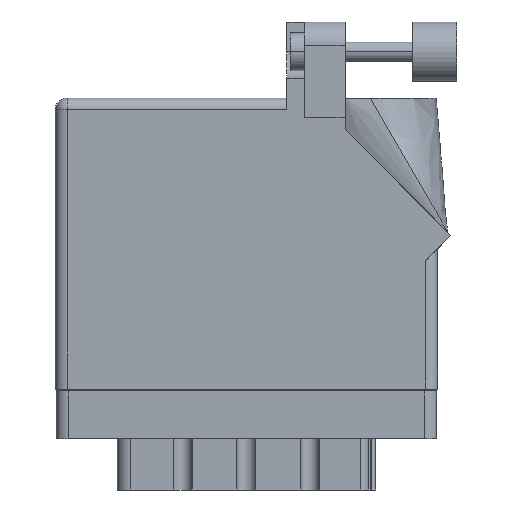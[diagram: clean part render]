
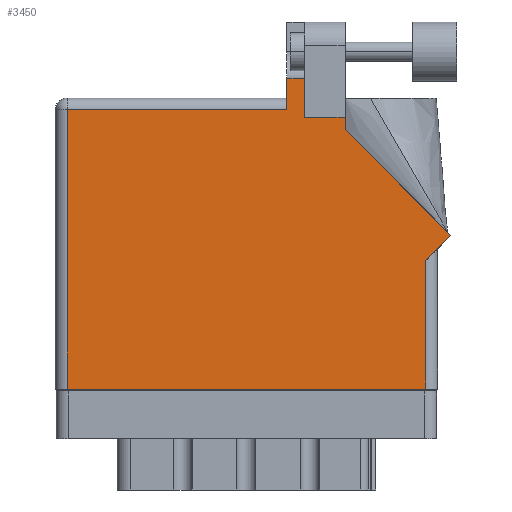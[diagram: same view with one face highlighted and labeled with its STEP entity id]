
A CAD part, front view. The second image highlights one B-rep face of the part: STEP entity #3450.
In plain terms, the highlighted face is planar.
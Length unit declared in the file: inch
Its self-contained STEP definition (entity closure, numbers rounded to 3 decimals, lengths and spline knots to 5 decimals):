
#1337 = CARTESIAN_POINT ( 'NONE',  ( 2.01, 0.737, 0. ) ) ;
#1990 = DIRECTION ( 'NONE',  ( 0., 0., -1. ) ) ;
#2199 = DIRECTION ( 'NONE',  ( 0., 1., 0. ) ) ;
#2645 = CARTESIAN_POINT ( 'NONE',  ( 1.311, 1.43, 0. ) ) ;
#2704 = VERTEX_POINT ( 'NONE', #9320 ) ;
#3338 = VECTOR ( 'NONE', #2199, 39.37008 ) ;
#3450 = ADVANCED_FACE ( 'NONE', ( #28694 ), #10248, .F. ) ;
#3927 = ORIENTED_EDGE ( 'NONE', *, *, #25449, .T. ) ;
#4566 = CARTESIAN_POINT ( 'NONE',  ( 1.311, 1.43, 0. ) ) ;
#4625 = LINE ( 'NONE', #37201, #21853 ) ;
#4755 = DIRECTION ( 'NONE',  ( -1., 0., 0. ) ) ;
#4997 = CARTESIAN_POINT ( 'NONE',  ( 1.524, 1.36442, 0. ) ) ;
#5608 = VERTEX_POINT ( 'NONE', #6258 ) ;
#6083 = EDGE_CURVE ( 'NONE', #9348, #12156, #30414, .T. ) ;
#6258 = CARTESIAN_POINT ( 'NONE',  ( 1.948, 0.675, 0. ) ) ;
#6453 = ORIENTED_EDGE ( 'NONE', *, *, #9667, .T. ) ;
#6529 = DIRECTION ( 'NONE',  ( 0., -1., 0. ) ) ;
#6634 = CARTESIAN_POINT ( 'NONE',  ( 1.524, 1.36442, 0. ) ) ;
#7300 = AXIS2_PLACEMENT_3D ( 'NONE', #19517, #1990, #31050 ) ;
#7605 = LINE ( 'NONE', #36098, #27580 ) ;
#7659 = CARTESIAN_POINT ( 'NONE',  ( 0., 1.468, 0. ) ) ;
#7669 = LINE ( 'NONE', #35610, #36247 ) ;
#8087 = ORIENTED_EDGE ( 'NONE', *, *, #18436, .T. ) ;
#8394 = CARTESIAN_POINT ( 'NONE',  ( 2.08071, 0.80771, 0. ) ) ;
#8496 = CARTESIAN_POINT ( 'NONE',  ( 1.217, 1.468, 0. ) ) ;
#9320 = CARTESIAN_POINT ( 'NONE',  ( 0.062, 1.468, 0. ) ) ;
#9348 = VERTEX_POINT ( 'NONE', #31632 ) ;
#9414 = CARTESIAN_POINT ( 'NONE',  ( 1.948, 0., 0. ) ) ;
#9667 = EDGE_CURVE ( 'NONE', #27981, #18224, #4625, .T. ) ;
#9725 = DIRECTION ( 'NONE',  ( 1., 0., 0. ) ) ;
#9809 = VERTEX_POINT ( 'NONE', #14018 ) ;
#9871 = DIRECTION ( 'NONE',  ( 0.707, 0.707, 0. ) ) ;
#10069 = ORIENTED_EDGE ( 'NONE', *, *, #20726, .T. ) ;
#10248 = PLANE ( 'NONE',  #7300 ) ;
#12108 = LINE ( 'NONE', #33736, #21128 ) ;
#12156 = VERTEX_POINT ( 'NONE', #6634 ) ;
#12233 = VERTEX_POINT ( 'NONE', #9414 ) ;
#12441 = VECTOR ( 'NONE', #34024, 39.37008 ) ;
#13345 = LINE ( 'NONE', #7659, #12441 ) ;
#14018 = CARTESIAN_POINT ( 'NONE',  ( 1.524, 1.43, 0. ) ) ;
#14030 = ORIENTED_EDGE ( 'NONE', *, *, #32396, .T. ) ;
#14276 = LINE ( 'NONE', #22393, #21044 ) ;
#15120 = CARTESIAN_POINT ( 'NONE',  ( 1.217, 1.6315, 0. ) ) ;
#16359 = DIRECTION ( 'NONE',  ( 0., 1., 0. ) ) ;
#16411 = EDGE_CURVE ( 'NONE', #22450, #12233, #32789, .T. ) ;
#18224 = VERTEX_POINT ( 'NONE', #8496 ) ;
#18436 = EDGE_CURVE ( 'NONE', #27429, #27981, #7669, .T. ) ;
#19517 = CARTESIAN_POINT ( 'NONE',  ( 0., 1.53, 0. ) ) ;
#19787 = DIRECTION ( 'NONE',  ( 0., 1., 0. ) ) ;
#20041 = DIRECTION ( 'NONE',  ( 0., -1., 0. ) ) ;
#20726 = EDGE_CURVE ( 'NONE', #2704, #22450, #7605, .T. ) ;
#21044 = VECTOR ( 'NONE', #22137, 39.37008 ) ;
#21128 = VECTOR ( 'NONE', #16359, 39.37008 ) ;
#21853 = VECTOR ( 'NONE', #20041, 39.37008 ) ;
#22137 = DIRECTION ( 'NONE',  ( -1., 0., 0. ) ) ;
#22393 = CARTESIAN_POINT ( 'NONE',  ( 1.524, 1.43, 0. ) ) ;
#22450 = VERTEX_POINT ( 'NONE', #26945 ) ;
#22606 = DIRECTION ( 'NONE',  ( -0.707, 0.707, 0. ) ) ;
#23024 = VECTOR ( 'NONE', #9871, 39.37008 ) ;
#23461 = LINE ( 'NONE', #1337, #23024 ) ;
#23972 = ORIENTED_EDGE ( 'NONE', *, *, #24792, .T. ) ;
#24242 = LINE ( 'NONE', #4997, #3338 ) ;
#24792 = EDGE_CURVE ( 'NONE', #12233, #5608, #12108, .T. ) ;
#25449 = EDGE_CURVE ( 'NONE', #12156, #9809, #24242, .T. ) ;
#25492 = ORIENTED_EDGE ( 'NONE', *, *, #16411, .T. ) ;
#25584 = ORIENTED_EDGE ( 'NONE', *, *, #29218, .T. ) ;
#25843 = VERTEX_POINT ( 'NONE', #4566 ) ;
#26328 = CARTESIAN_POINT ( 'NONE',  ( 1.311, 1.6315, 0. ) ) ;
#26468 = VECTOR ( 'NONE', #9725, 39.37008 ) ;
#26716 = ORIENTED_EDGE ( 'NONE', *, *, #31774, .T. ) ;
#26945 = CARTESIAN_POINT ( 'NONE',  ( 0.062, 0., 0. ) ) ;
#27258 = ORIENTED_EDGE ( 'NONE', *, *, #6083, .T. ) ;
#27429 = VERTEX_POINT ( 'NONE', #26328 ) ;
#27580 = VECTOR ( 'NONE', #6529, 39.37008 ) ;
#27981 = VERTEX_POINT ( 'NONE', #15120 ) ;
#28694 = FACE_OUTER_BOUND ( 'NONE', #32839, .T. ) ;
#29218 = EDGE_CURVE ( 'NONE', #5608, #9348, #23461, .T. ) ;
#30400 = CARTESIAN_POINT ( 'NONE',  ( 0., 0., 0. ) ) ;
#30414 = LINE ( 'NONE', #8394, #36334 ) ;
#31050 = DIRECTION ( 'NONE',  ( -1., 0., 0. ) ) ;
#31632 = CARTESIAN_POINT ( 'NONE',  ( 2.08071, 0.80771, 0. ) ) ;
#31774 = EDGE_CURVE ( 'NONE', #18224, #2704, #13345, .T. ) ;
#32304 = ORIENTED_EDGE ( 'NONE', *, *, #34923, .T. ) ;
#32396 = EDGE_CURVE ( 'NONE', #25843, #27429, #37551, .T. ) ;
#32789 = LINE ( 'NONE', #30400, #26468 ) ;
#32839 = EDGE_LOOP ( 'NONE', ( #14030, #8087, #6453, #26716, #10069, #25492, #23972, #25584, #27258, #3927, #32304 ) ) ;
#33736 = CARTESIAN_POINT ( 'NONE',  ( 1.948, 0.737, 0. ) ) ;
#34024 = DIRECTION ( 'NONE',  ( -1., 0., 0. ) ) ;
#34923 = EDGE_CURVE ( 'NONE', #9809, #25843, #14276, .T. ) ;
#35610 = CARTESIAN_POINT ( 'NONE',  ( 1.64177, 1.6315, 0. ) ) ;
#36098 = CARTESIAN_POINT ( 'NONE',  ( 0.062, 0., 0. ) ) ;
#36186 = VECTOR ( 'NONE', #19787, 39.37008 ) ;
#36247 = VECTOR ( 'NONE', #4755, 39.37008 ) ;
#36334 = VECTOR ( 'NONE', #22606, 39.37008 ) ;
#37201 = CARTESIAN_POINT ( 'NONE',  ( 1.217, 1.53, 0. ) ) ;
#37551 = LINE ( 'NONE', #2645, #36186 ) ;
